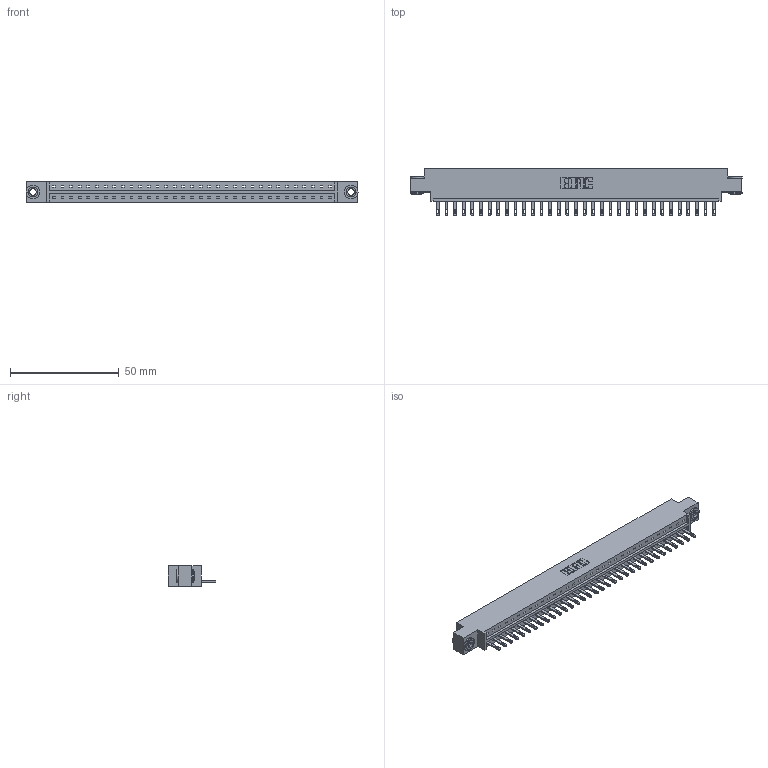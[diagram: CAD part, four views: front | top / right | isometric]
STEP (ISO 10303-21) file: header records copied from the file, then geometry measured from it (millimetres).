
FILE_DESCRIPTION (( 'STEP AP203' ), '1' );
FILE_NAME ('833-033-500-603.STEP', '2020-06-02T19:41:52', ( '' ), ( '' ), 'SwSTEP 2.0', 'SolidWorks 2020', '' );
FILE_SCHEMA (( 'CONFIG_CONTROL_DESIGN' ));
Length unit declared in the file: inch
Products named in the file (4): 833-033-500-603; 833 Part_Offset - .156 Dia - TH; 345-292-001_345-293-100; 345-250-002_345-250-002-102
Assembly tree (36 placements, depth 2):
  833-033-500-603
    833 Part_Offset - .156 Dia - TH
    345-292-001_345-293-100  x33
    345-250-002_345-250-002-102  x2
Bounding box: 152.3 x 21.85 x 9.4 mm (x, y, z)
Volume: 15060.1 mm3; surface area: 16741.6 mm2
Topology: 36 solids, 36 shells, 1938 faces, 5943 edges, 3958 vertices
Faces by surface type: plane 1272, cylinder 658, cone 8
Entity records: 22050 total; most frequent: CARTESIAN_POINT 3784, ORIENTED_EDGE 3746, DIRECTION 3245, EDGE_CURVE 1873, LINE 1717, VECTOR 1717, VERTEX_POINT 1246, AXIS2_PLACEMENT_3D 764
